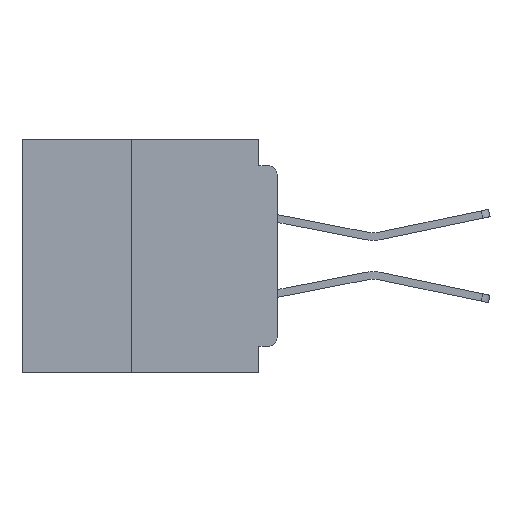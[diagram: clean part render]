
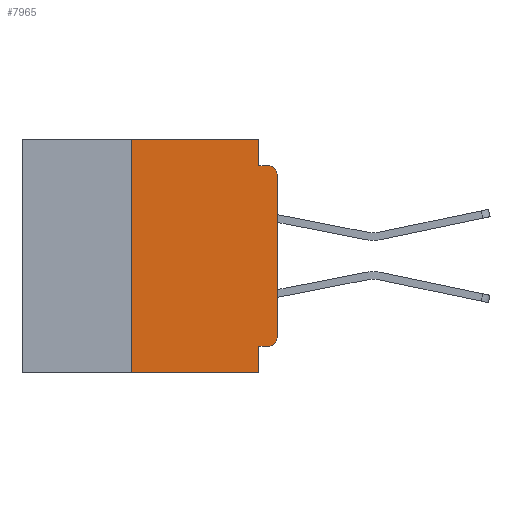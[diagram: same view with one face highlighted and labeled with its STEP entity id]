
A CAD part, left-side view. The second image highlights one B-rep face of the part: STEP entity #7965.
In plain terms, the highlighted planar face has unit normal (-1, 0, 0).
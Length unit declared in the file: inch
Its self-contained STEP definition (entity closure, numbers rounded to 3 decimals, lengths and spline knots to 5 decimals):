
#913 = LINE ( 'NONE', #52011, #43314 ) ;
#948 = CARTESIAN_POINT ( 'NONE',  ( 0., 0., -0.06 ) ) ;
#1618 = LINE ( 'NONE', #43603, #23707 ) ;
#1865 = ORIENTED_EDGE ( 'NONE', *, *, #4417, .F. ) ;
#2236 = EDGE_CURVE ( 'NONE', #31353, #4853, #36329, .T. ) ;
#4005 = ORIENTED_EDGE ( 'NONE', *, *, #55875, .F. ) ;
#4326 = CARTESIAN_POINT ( 'NONE',  ( 0., 0., -0.045 ) ) ;
#4417 = EDGE_CURVE ( 'NONE', #54518, #32595, #30076, .T. ) ;
#4631 = DIRECTION ( 'NONE',  ( -1., 0., 0. ) ) ;
#4853 = VERTEX_POINT ( 'NONE', #7579 ) ;
#5849 = CARTESIAN_POINT ( 'NONE',  ( 0., 0.031, -0.4 ) ) ;
#6299 = EDGE_CURVE ( 'NONE', #32595, #54495, #913, .T. ) ;
#7579 = CARTESIAN_POINT ( 'NONE',  ( 0., 0.031, -0.045 ) ) ;
#7965 = ADVANCED_FACE ( 'NONE', ( #19331 ), #33233, .F. ) ;
#8040 = VECTOR ( 'NONE', #10867, 39.37008 ) ;
#8505 = ORIENTED_EDGE ( 'NONE', *, *, #29897, .T. ) ;
#8703 = AXIS2_PLACEMENT_3D ( 'NONE', #36750, #10521, #41056 ) ;
#8980 = VECTOR ( 'NONE', #33764, 39.37008 ) ;
#10521 = DIRECTION ( 'NONE',  ( -1., 0., 0. ) ) ;
#10867 = DIRECTION ( 'NONE',  ( 0., 0., 1. ) ) ;
#11277 = LINE ( 'NONE', #4326, #56124 ) ;
#11537 = DIRECTION ( 'NONE',  ( 1., 0., 0. ) ) ;
#11781 = CARTESIAN_POINT ( 'NONE',  ( 0., 0.031, -0.355 ) ) ;
#12460 = CARTESIAN_POINT ( 'NONE',  ( 0., 0., -0.355 ) ) ;
#13408 = DIRECTION ( 'NONE',  ( 0., -1., 0. ) ) ;
#13431 = ORIENTED_EDGE ( 'NONE', *, *, #2236, .F. ) ;
#14061 = EDGE_CURVE ( 'NONE', #38279, #28219, #44221, .T. ) ;
#16144 = CARTESIAN_POINT ( 'NONE',  ( 0., 0.031, 0. ) ) ;
#16943 = CIRCLE ( 'NONE', #8703, 0.015 ) ;
#18973 = VERTEX_POINT ( 'NONE', #53370 ) ;
#19331 = FACE_OUTER_BOUND ( 'NONE', #42438, .T. ) ;
#20433 = DIRECTION ( 'NONE',  ( 0., 0., -1. ) ) ;
#20617 = CARTESIAN_POINT ( 'NONE',  ( 0., 0.031, 0. ) ) ;
#21802 = CARTESIAN_POINT ( 'NONE',  ( 0., 0., -0.34 ) ) ;
#22031 = VECTOR ( 'NONE', #20433, 39.37008 ) ;
#23425 = ORIENTED_EDGE ( 'NONE', *, *, #14061, .T. ) ;
#23707 = VECTOR ( 'NONE', #47950, 39.37008 ) ;
#26140 = DIRECTION ( 'NONE',  ( 0., 0., -1. ) ) ;
#26227 = EDGE_CURVE ( 'NONE', #28219, #44833, #16943, .T. ) ;
#28115 = CARTESIAN_POINT ( 'NONE',  ( 0., 0.015, -0.045 ) ) ;
#28219 = VERTEX_POINT ( 'NONE', #948 ) ;
#28387 = CARTESIAN_POINT ( 'NONE',  ( 0., 0., 0. ) ) ;
#29380 = CARTESIAN_POINT ( 'NONE',  ( 0., 0.437, 0. ) ) ;
#29402 = CARTESIAN_POINT ( 'NONE',  ( 0., 0.25, -0.4 ) ) ;
#29897 = EDGE_CURVE ( 'NONE', #47173, #54495, #1618, .T. ) ;
#30076 = LINE ( 'NONE', #12460, #41525 ) ;
#30601 = AXIS2_PLACEMENT_3D ( 'NONE', #31006, #4631, #35331 ) ;
#30969 = VECTOR ( 'NONE', #42368, 39.37008 ) ;
#31006 = CARTESIAN_POINT ( 'NONE',  ( 0., 0.015, -0.34 ) ) ;
#31353 = VERTEX_POINT ( 'NONE', #16144 ) ;
#31473 = CIRCLE ( 'NONE', #30601, 0.015 ) ;
#32395 = CARTESIAN_POINT ( 'NONE',  ( 0., 0.015, -0.355 ) ) ;
#32595 = VERTEX_POINT ( 'NONE', #11781 ) ;
#33233 = PLANE ( 'NONE',  #46264 ) ;
#33764 = DIRECTION ( 'NONE',  ( 0., 0., 1. ) ) ;
#35331 = DIRECTION ( 'NONE',  ( 0., 0., -1. ) ) ;
#35972 = ORIENTED_EDGE ( 'NONE', *, *, #43631, .F. ) ;
#36329 = LINE ( 'NONE', #20617, #22031 ) ;
#36750 = CARTESIAN_POINT ( 'NONE',  ( 0., 0.015, -0.06 ) ) ;
#37718 = CARTESIAN_POINT ( 'NONE',  ( 0., 0.437, 0. ) ) ;
#38279 = VERTEX_POINT ( 'NONE', #21802 ) ;
#39614 = EDGE_CURVE ( 'NONE', #4853, #44833, #11277, .T. ) ;
#41056 = DIRECTION ( 'NONE',  ( 0., 0., -1. ) ) ;
#41525 = VECTOR ( 'NONE', #47276, 39.37008 ) ;
#42027 = DIRECTION ( 'NONE',  ( 0., 0., -1. ) ) ;
#42368 = DIRECTION ( 'NONE',  ( 0., -1., 0. ) ) ;
#42438 = EDGE_LOOP ( 'NONE', ( #23425, #51019, #43456, #13431, #35972, #4005, #8505, #54686, #1865, #56440 ) ) ;
#43314 = VECTOR ( 'NONE', #26140, 39.37008 ) ;
#43456 = ORIENTED_EDGE ( 'NONE', *, *, #39614, .F. ) ;
#43603 = CARTESIAN_POINT ( 'NONE',  ( 0., 0.437, -0.4 ) ) ;
#43631 = EDGE_CURVE ( 'NONE', #18973, #31353, #53844, .T. ) ;
#43773 = LINE ( 'NONE', #29402, #8980 ) ;
#44221 = LINE ( 'NONE', #28387, #8040 ) ;
#44833 = VERTEX_POINT ( 'NONE', #28115 ) ;
#46264 = AXIS2_PLACEMENT_3D ( 'NONE', #37718, #11537, #42027 ) ;
#47173 = VERTEX_POINT ( 'NONE', #48998 ) ;
#47276 = DIRECTION ( 'NONE',  ( 0., 1., 0. ) ) ;
#47950 = DIRECTION ( 'NONE',  ( 0., -1., 0. ) ) ;
#48998 = CARTESIAN_POINT ( 'NONE',  ( 0., 0.25, -0.4 ) ) ;
#50450 = EDGE_CURVE ( 'NONE', #54518, #38279, #31473, .T. ) ;
#51019 = ORIENTED_EDGE ( 'NONE', *, *, #26227, .T. ) ;
#52011 = CARTESIAN_POINT ( 'NONE',  ( 0., 0.031, -0.4 ) ) ;
#53370 = CARTESIAN_POINT ( 'NONE',  ( 0., 0.25, 0. ) ) ;
#53844 = LINE ( 'NONE', #29380, #30969 ) ;
#54495 = VERTEX_POINT ( 'NONE', #5849 ) ;
#54518 = VERTEX_POINT ( 'NONE', #32395 ) ;
#54686 = ORIENTED_EDGE ( 'NONE', *, *, #6299, .F. ) ;
#55875 = EDGE_CURVE ( 'NONE', #47173, #18973, #43773, .T. ) ;
#56124 = VECTOR ( 'NONE', #13408, 39.37008 ) ;
#56440 = ORIENTED_EDGE ( 'NONE', *, *, #50450, .T. ) ;
